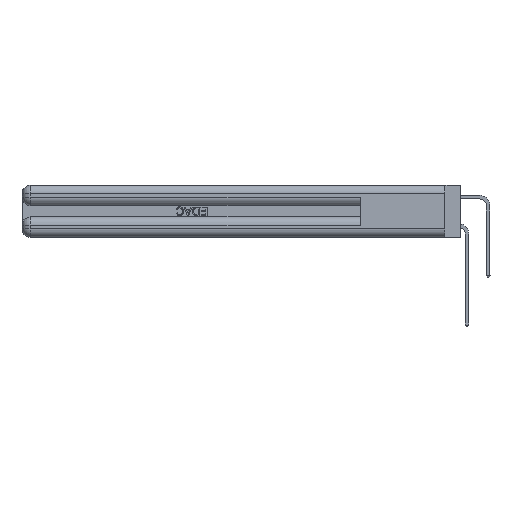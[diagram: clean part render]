
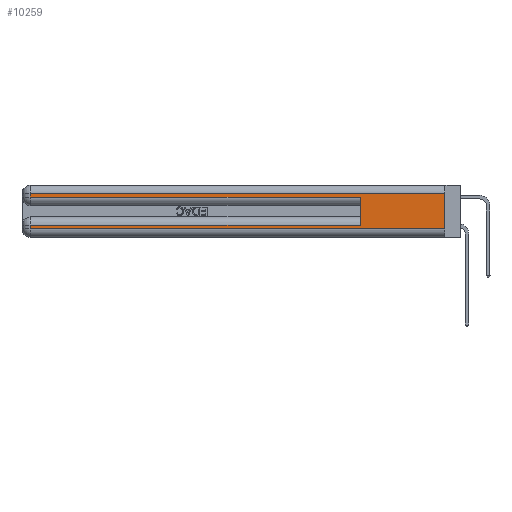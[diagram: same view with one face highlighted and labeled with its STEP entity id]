
A CAD part, left-side view. The second image highlights one B-rep face of the part: STEP entity #10259.
In plain terms, the highlighted planar face has unit normal (-1, 0, 0).
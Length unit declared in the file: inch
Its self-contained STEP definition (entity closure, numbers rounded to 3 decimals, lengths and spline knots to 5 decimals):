
#833 = DIRECTION ( 'NONE',  ( 0., 0., -1. ) ) ;
#1483 = LINE ( 'NONE', #45300, #40492 ) ;
#1637 = DIRECTION ( 'NONE',  ( 0., 0., -1. ) ) ;
#1655 = LINE ( 'NONE', #21122, #39448 ) ;
#2031 = LINE ( 'NONE', #11098, #42222 ) ;
#2877 = VERTEX_POINT ( 'NONE', #5378 ) ;
#3030 = ORIENTED_EDGE ( 'NONE', *, *, #49881, .T. ) ;
#3392 = DIRECTION ( 'NONE',  ( 0., -1., 0. ) ) ;
#3667 = CARTESIAN_POINT ( 'NONE',  ( 0., 0.6, 0.085 ) ) ;
#5267 = CARTESIAN_POINT ( 'NONE',  ( 0., 0., 0.31 ) ) ;
#5378 = CARTESIAN_POINT ( 'NONE',  ( 0., 2.94, 0.31 ) ) ;
#5745 = ORIENTED_EDGE ( 'NONE', *, *, #35340, .F. ) ;
#6388 = ORIENTED_EDGE ( 'NONE', *, *, #29426, .T. ) ;
#7518 = LINE ( 'NONE', #47430, #46395 ) ;
#8457 = EDGE_CURVE ( 'NONE', #40103, #39251, #2031, .T. ) ;
#9500 = EDGE_CURVE ( 'NONE', #35226, #44758, #28189, .T. ) ;
#9533 = VERTEX_POINT ( 'NONE', #3667 ) ;
#10259 = ADVANCED_FACE ( 'NONE', ( #32958 ), #31223, .F. ) ;
#10659 = DIRECTION ( 'NONE',  ( 0., 1., 0. ) ) ;
#11098 = CARTESIAN_POINT ( 'NONE',  ( 0., 0., 0.06 ) ) ;
#11803 = DIRECTION ( 'NONE',  ( 1., 0., 0. ) ) ;
#14184 = ORIENTED_EDGE ( 'NONE', *, *, #8457, .T. ) ;
#18786 = CARTESIAN_POINT ( 'NONE',  ( 0., 0., 0.06 ) ) ;
#18818 = CARTESIAN_POINT ( 'NONE',  ( 0., 0.6, 0.145 ) ) ;
#19243 = EDGE_CURVE ( 'NONE', #9533, #41590, #1483, .T. ) ;
#19779 = ORIENTED_EDGE ( 'NONE', *, *, #47543, .F. ) ;
#20778 = VECTOR ( 'NONE', #42041, 39.37008 ) ;
#21122 = CARTESIAN_POINT ( 'NONE',  ( 0., 0., 0.37 ) ) ;
#21292 = CARTESIAN_POINT ( 'NONE',  ( 0., 2.94, 0.085 ) ) ;
#21836 = VERTEX_POINT ( 'NONE', #5267 ) ;
#25174 = VECTOR ( 'NONE', #50185, 39.37008 ) ;
#25724 = ORIENTED_EDGE ( 'NONE', *, *, #9500, .T. ) ;
#27677 = LINE ( 'NONE', #49117, #45819 ) ;
#28189 = LINE ( 'NONE', #45981, #47528 ) ;
#29079 = EDGE_LOOP ( 'NONE', ( #19779, #3030, #33111, #25724, #5745, #42047, #6388, #14184 ) ) ;
#29426 = EDGE_CURVE ( 'NONE', #41590, #40103, #7518, .T. ) ;
#29890 = DIRECTION ( 'NONE',  ( 0., 1., 0. ) ) ;
#30808 = CARTESIAN_POINT ( 'NONE',  ( 0., 2.94, 0.37 ) ) ;
#31223 = PLANE ( 'NONE',  #39886 ) ;
#31430 = CARTESIAN_POINT ( 'NONE',  ( 0., 2.94, 0.06 ) ) ;
#32958 = FACE_OUTER_BOUND ( 'NONE', #29079, .T. ) ;
#33111 = ORIENTED_EDGE ( 'NONE', *, *, #34169, .T. ) ;
#34169 = EDGE_CURVE ( 'NONE', #2877, #35226, #35501, .T. ) ;
#35121 = CARTESIAN_POINT ( 'NONE',  ( 0., 0., 0.37 ) ) ;
#35226 = VERTEX_POINT ( 'NONE', #49102 ) ;
#35340 = EDGE_CURVE ( 'NONE', #9533, #44758, #41438, .T. ) ;
#35501 = LINE ( 'NONE', #30808, #25174 ) ;
#39032 = DIRECTION ( 'NONE',  ( 0., 0., -1. ) ) ;
#39251 = VERTEX_POINT ( 'NONE', #18786 ) ;
#39448 = VECTOR ( 'NONE', #1637, 39.37008 ) ;
#39886 = AXIS2_PLACEMENT_3D ( 'NONE', #35121, #11803, #39032 ) ;
#40103 = VERTEX_POINT ( 'NONE', #31430 ) ;
#40492 = VECTOR ( 'NONE', #10659, 39.37008 ) ;
#41438 = LINE ( 'NONE', #18818, #20778 ) ;
#41590 = VERTEX_POINT ( 'NONE', #21292 ) ;
#42041 = DIRECTION ( 'NONE',  ( 0., 0., 1. ) ) ;
#42047 = ORIENTED_EDGE ( 'NONE', *, *, #19243, .T. ) ;
#42222 = VECTOR ( 'NONE', #3392, 39.37008 ) ;
#44758 = VERTEX_POINT ( 'NONE', #47220 ) ;
#45300 = CARTESIAN_POINT ( 'NONE',  ( 0., 0., 0.085 ) ) ;
#45819 = VECTOR ( 'NONE', #29890, 39.37008 ) ;
#45981 = CARTESIAN_POINT ( 'NONE',  ( 0., 0., 0.285 ) ) ;
#46395 = VECTOR ( 'NONE', #833, 39.37008 ) ;
#47220 = CARTESIAN_POINT ( 'NONE',  ( 0., 0.6, 0.285 ) ) ;
#47430 = CARTESIAN_POINT ( 'NONE',  ( 0., 2.94, 0.37 ) ) ;
#47528 = VECTOR ( 'NONE', #49847, 39.37008 ) ;
#47543 = EDGE_CURVE ( 'NONE', #21836, #39251, #1655, .T. ) ;
#49102 = CARTESIAN_POINT ( 'NONE',  ( 0., 2.94, 0.285 ) ) ;
#49117 = CARTESIAN_POINT ( 'NONE',  ( 0., 0., 0.31 ) ) ;
#49847 = DIRECTION ( 'NONE',  ( 0., -1., 0. ) ) ;
#49881 = EDGE_CURVE ( 'NONE', #21836, #2877, #27677, .T. ) ;
#50185 = DIRECTION ( 'NONE',  ( 0., 0., -1. ) ) ;
